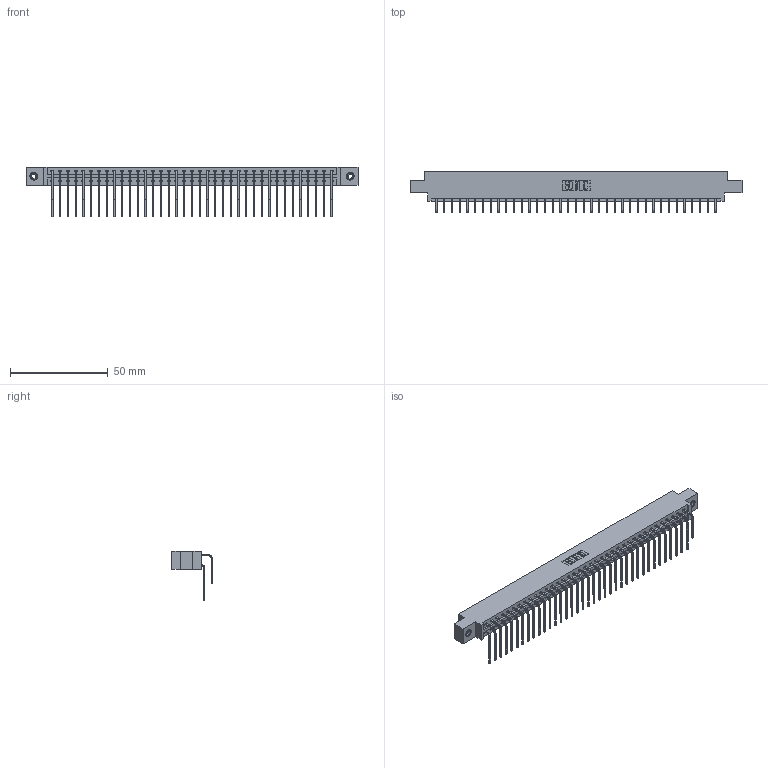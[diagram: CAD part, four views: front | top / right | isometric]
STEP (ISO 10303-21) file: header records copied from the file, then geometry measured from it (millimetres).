
FILE_DESCRIPTION (( 'STEP AP203' ), '1' );
FILE_NAME ('387-074-559-808.STEP', '2019-10-22T02:41:45', ( '' ), ( '' ), 'SwSTEP 2.0', 'SolidWorks 2016', '' );
FILE_SCHEMA (( 'CONFIG_CONTROL_DESIGN' ));
Length unit declared in the file: inch
Products named in the file (5): 345-250-001_345-250-003-102; 345-292-001_559 Tail - 2; 345-292-001_558 559 Tail - 1; 387-074-559-808; 337 Part_0.170 Offset - 0.156 Dia-TI
Assembly tree (77 placements, depth 2):
  387-074-559-808
    337 Part_0.170 Offset - 0.156 Dia-TI
    345-292-001_558 559 Tail - 1  x37
    345-292-001_559 Tail - 2  x37
    345-250-001_345-250-003-102  x2
Bounding box: 169.62 x 20.9 x 25.53 mm (x, y, z)
Volume: 18112.3 mm3; surface area: 22702.7 mm2
Topology: 77 solids, 77 shells, 4322 faces, 12817 edges, 8438 vertices
Faces by surface type: plane 3066, cylinder 1240, cone 12, torus 4
Entity records: 32436 total; most frequent: CARTESIAN_POINT 5496, ORIENTED_EDGE 5374, DIRECTION 4697, EDGE_CURVE 2687, LINE 2499, VECTOR 2499, VERTEX_POINT 1784, AXIS2_PLACEMENT_3D 1099
